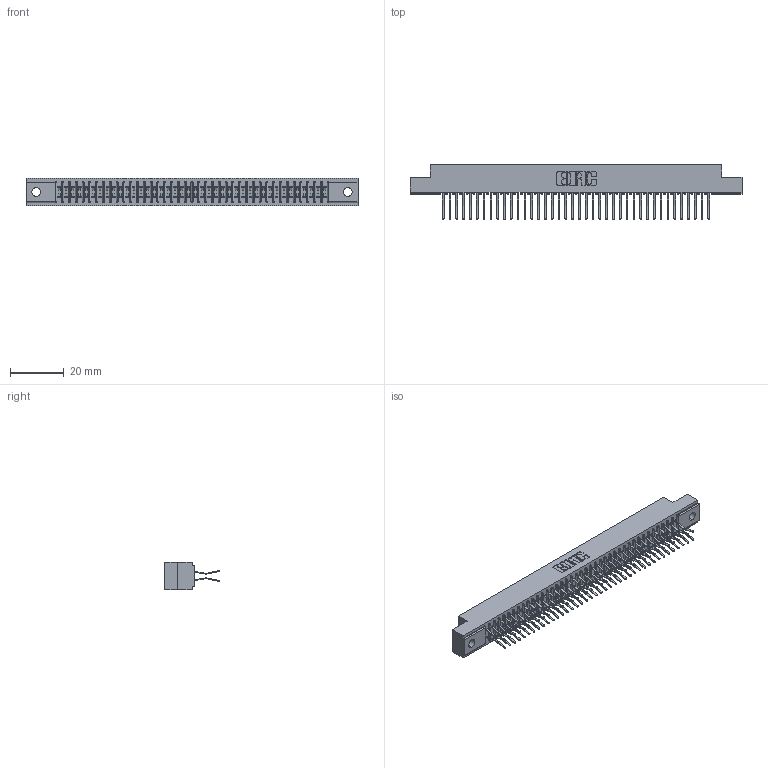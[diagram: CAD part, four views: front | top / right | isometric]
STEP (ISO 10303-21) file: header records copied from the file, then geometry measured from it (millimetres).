
FILE_DESCRIPTION (( 'STEP AP203' ), '1' );
FILE_NAME ('341-080-560-202.STEP', '2018-08-07T21:55:16', ( '' ), ( '' ), 'SwSTEP 2.0', 'SolidWorks 2016', '' );
FILE_SCHEMA (( 'CONFIG_CONTROL_DESIGN' ));
Length unit declared in the file: inch
Products named in the file (3): 341-292-001_341-292-160; 341-080-560-202; 341 Part_.128 (3.25) Dia Mounting Holes
Assembly tree (81 placements, depth 2):
  341-080-560-202
    341 Part_.128 (3.25) Dia Mounting Holes
    341-292-001_341-292-160  x80
Bounding box: 123.83 x 20.37 x 10.16 mm (x, y, z)
Volume: 9181.4 mm3; surface area: 16576.3 mm2
Topology: 81 solids, 81 shells, 5716 faces, 16596 edges, 10766 vertices
Faces by surface type: plane 3268, cylinder 2288, sphere 82, torus 78
Entity records: 48817 total; most frequent: CARTESIAN_POINT 8116, ORIENTED_EDGE 8064, DIRECTION 7882, EDGE_CURVE 4032, VECTOR 3250, LINE 3250, VERTEX_POINT 2550, AXIS2_PLACEMENT_3D 2316
